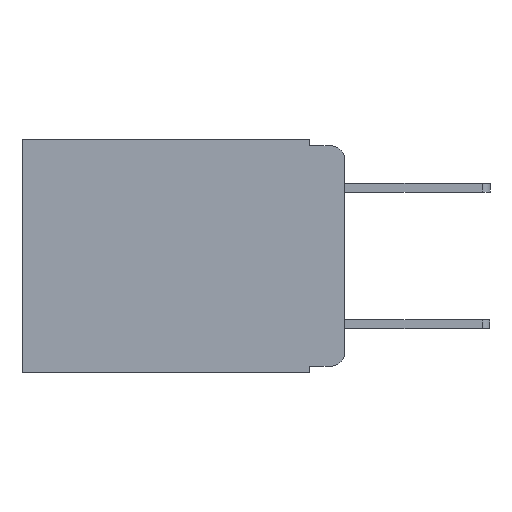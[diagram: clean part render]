
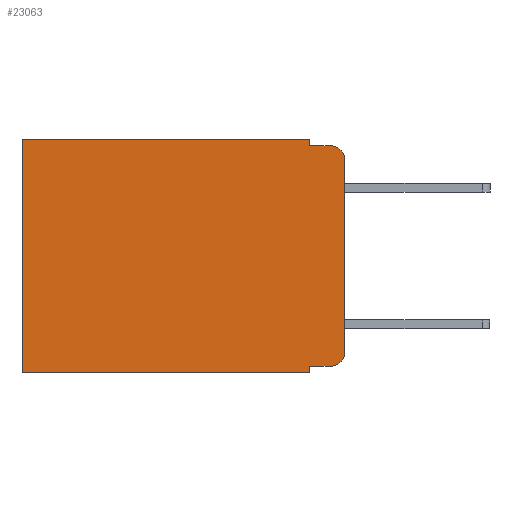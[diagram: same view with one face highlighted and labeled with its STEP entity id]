
A CAD part, left-side view. The second image highlights one B-rep face of the part: STEP entity #23063.
In plain terms, the highlighted planar face has unit normal (-1, 0, 0).
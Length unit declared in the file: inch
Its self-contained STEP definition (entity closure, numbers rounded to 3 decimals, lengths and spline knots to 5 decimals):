
#52 = CARTESIAN_POINT ( 'NONE',  ( 0.298, 0., -0.343 ) ) ;
#62 = LINE ( 'NONE', #3339, #9564 ) ;
#1272 = CARTESIAN_POINT ( 'NONE',  ( 0.298, 0., -0.313 ) ) ;
#1299 = VECTOR ( 'NONE', #3959, 39.37008 ) ;
#1321 = DIRECTION ( 'NONE',  ( 0., 1., 0. ) ) ;
#1410 = ORIENTED_EDGE ( 'NONE', *, *, #14364, .T. ) ;
#1450 = DIRECTION ( 'NONE',  ( 0., -1., 0. ) ) ;
#1587 = CARTESIAN_POINT ( 'NONE',  ( 0.298, 0.051, 0. ) ) ;
#2261 = VERTEX_POINT ( 'NONE', #1587 ) ;
#2435 = EDGE_CURVE ( 'NONE', #14314, #17262, #62, .T. ) ;
#2502 = CARTESIAN_POINT ( 'NONE',  ( 0.298, 0.051, 0. ) ) ;
#2920 = CARTESIAN_POINT ( 'NONE',  ( 0.298, 0.051, -0.343 ) ) ;
#3339 = CARTESIAN_POINT ( 'NONE',  ( 0.298, 0.051, 0. ) ) ;
#3632 = DIRECTION ( 'NONE',  ( 0., -1., 0. ) ) ;
#3701 = VECTOR ( 'NONE', #1321, 39.37008 ) ;
#3959 = DIRECTION ( 'NONE',  ( 0., 0., -1. ) ) ;
#4024 = DIRECTION ( 'NONE',  ( 1., 0., 0. ) ) ;
#4221 = ORIENTED_EDGE ( 'NONE', *, *, #23441, .T. ) ;
#4381 = DIRECTION ( 'NONE',  ( -1., 0., 0. ) ) ;
#5104 = ORIENTED_EDGE ( 'NONE', *, *, #2435, .F. ) ;
#5159 = VERTEX_POINT ( 'NONE', #5323 ) ;
#5323 = CARTESIAN_POINT ( 'NONE',  ( 0.298, 0.473, -0.343 ) ) ;
#5409 = LINE ( 'NONE', #52, #10897 ) ;
#5478 = EDGE_CURVE ( 'NONE', #7521, #5159, #18933, .T. ) ;
#5614 = VERTEX_POINT ( 'NONE', #17766 ) ;
#7042 = EDGE_CURVE ( 'NONE', #5614, #15538, #20224, .T. ) ;
#7061 = ORIENTED_EDGE ( 'NONE', *, *, #16745, .T. ) ;
#7346 = ORIENTED_EDGE ( 'NONE', *, *, #18077, .F. ) ;
#7395 = VECTOR ( 'NONE', #1450, 39.37008 ) ;
#7521 = VERTEX_POINT ( 'NONE', #14085 ) ;
#8156 = LINE ( 'NONE', #12505, #3701 ) ;
#8364 = FACE_OUTER_BOUND ( 'NONE', #9687, .T. ) ;
#8542 = ORIENTED_EDGE ( 'NONE', *, *, #19008, .T. ) ;
#8989 = CARTESIAN_POINT ( 'NONE',  ( 0.298, 0.051, -0.333 ) ) ;
#9404 = AXIS2_PLACEMENT_3D ( 'NONE', #15031, #4024, #16820 ) ;
#9564 = VECTOR ( 'NONE', #11960, 39.37008 ) ;
#9569 = EDGE_CURVE ( 'NONE', #17262, #5159, #5409, .T. ) ;
#9687 = EDGE_LOOP ( 'NONE', ( #11057, #4221, #14715, #7346, #7061, #16509, #20092, #5104, #1410, #8542 ) ) ;
#10705 = VERTEX_POINT ( 'NONE', #1272 ) ;
#10734 = VECTOR ( 'NONE', #3632, 39.37008 ) ;
#10897 = VECTOR ( 'NONE', #13142, 39.37008 ) ;
#11057 = ORIENTED_EDGE ( 'NONE', *, *, #16400, .F. ) ;
#11197 = CARTESIAN_POINT ( 'NONE',  ( 0.298, 0.02, -0.313 ) ) ;
#11278 = LINE ( 'NONE', #16760, #1299 ) ;
#11782 = DIRECTION ( 'NONE',  ( 0., 0., -1. ) ) ;
#11960 = DIRECTION ( 'NONE',  ( 0., 0., -1. ) ) ;
#12505 = CARTESIAN_POINT ( 'NONE',  ( 0.298, 0., 0. ) ) ;
#12790 = LINE ( 'NONE', #8989, #7395 ) ;
#13012 = DIRECTION ( 'NONE',  ( 0., 0., -1. ) ) ;
#13142 = DIRECTION ( 'NONE',  ( 0., 1., 0. ) ) ;
#14085 = CARTESIAN_POINT ( 'NONE',  ( 0.298, 0.473, 0. ) ) ;
#14314 = VERTEX_POINT ( 'NONE', #21294 ) ;
#14364 = EDGE_CURVE ( 'NONE', #14314, #16993, #12790, .T. ) ;
#14715 = ORIENTED_EDGE ( 'NONE', *, *, #7042, .F. ) ;
#14998 = AXIS2_PLACEMENT_3D ( 'NONE', #15351, #4381, #17133 ) ;
#15031 = CARTESIAN_POINT ( 'NONE',  ( 0.298, 0., 0. ) ) ;
#15169 = CIRCLE ( 'NONE', #14998, 0.02 ) ;
#15247 = VECTOR ( 'NONE', #11782, 39.37008 ) ;
#15351 = CARTESIAN_POINT ( 'NONE',  ( 0.298, 0.02, -0.03 ) ) ;
#15538 = VERTEX_POINT ( 'NONE', #18023 ) ;
#16378 = CARTESIAN_POINT ( 'NONE',  ( 0.298, 0.051, -0.01 ) ) ;
#16400 = EDGE_CURVE ( 'NONE', #16433, #10705, #11278, .T. ) ;
#16433 = VERTEX_POINT ( 'NONE', #20446 ) ;
#16509 = ORIENTED_EDGE ( 'NONE', *, *, #5478, .T. ) ;
#16745 = EDGE_CURVE ( 'NONE', #2261, #7521, #8156, .T. ) ;
#16760 = CARTESIAN_POINT ( 'NONE',  ( 0.298, 0., 0. ) ) ;
#16820 = DIRECTION ( 'NONE',  ( 0., 0., -1. ) ) ;
#16993 = VERTEX_POINT ( 'NONE', #20272 ) ;
#17092 = DIRECTION ( 'NONE',  ( 0., 0., -1. ) ) ;
#17133 = DIRECTION ( 'NONE',  ( 0., 0., -1. ) ) ;
#17262 = VERTEX_POINT ( 'NONE', #2920 ) ;
#17312 = AXIS2_PLACEMENT_3D ( 'NONE', #11197, #23572, #13012 ) ;
#17766 = CARTESIAN_POINT ( 'NONE',  ( 0.298, 0.051, -0.01 ) ) ;
#18023 = CARTESIAN_POINT ( 'NONE',  ( 0.298, 0.02, -0.01 ) ) ;
#18077 = EDGE_CURVE ( 'NONE', #2261, #5614, #19946, .T. ) ;
#18366 = VECTOR ( 'NONE', #17092, 39.37008 ) ;
#18860 = CARTESIAN_POINT ( 'NONE',  ( 0.298, 0.473, 0. ) ) ;
#18933 = LINE ( 'NONE', #18860, #18366 ) ;
#19008 = EDGE_CURVE ( 'NONE', #16993, #10705, #21784, .T. ) ;
#19946 = LINE ( 'NONE', #2502, #15247 ) ;
#20092 = ORIENTED_EDGE ( 'NONE', *, *, #9569, .F. ) ;
#20224 = LINE ( 'NONE', #16378, #10734 ) ;
#20272 = CARTESIAN_POINT ( 'NONE',  ( 0.298, 0.02, -0.333 ) ) ;
#20278 = PLANE ( 'NONE',  #9404 ) ;
#20446 = CARTESIAN_POINT ( 'NONE',  ( 0.298, 0., -0.03 ) ) ;
#21294 = CARTESIAN_POINT ( 'NONE',  ( 0.298, 0.051, -0.333 ) ) ;
#21784 = CIRCLE ( 'NONE', #17312, 0.02 ) ;
#23063 = ADVANCED_FACE ( 'NONE', ( #8364 ), #20278, .F. ) ;
#23441 = EDGE_CURVE ( 'NONE', #16433, #15538, #15169, .T. ) ;
#23572 = DIRECTION ( 'NONE',  ( -1., 0., 0. ) ) ;
